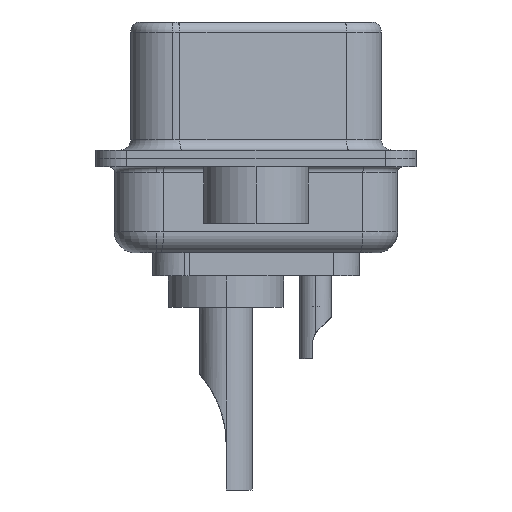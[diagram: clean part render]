
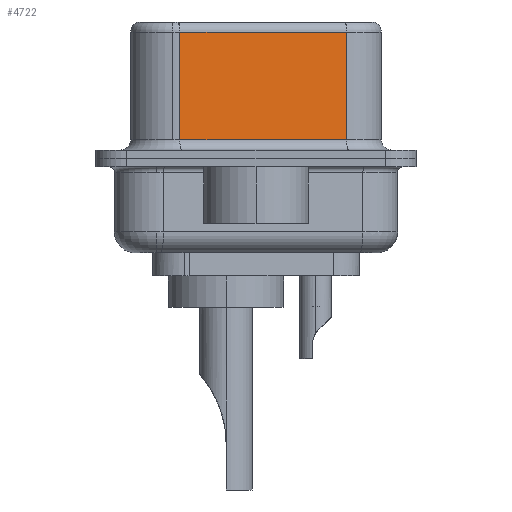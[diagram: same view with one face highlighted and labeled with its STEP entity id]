
A CAD part, left-side view. The second image highlights one B-rep face of the part: STEP entity #4722.
In plain terms, the highlighted planar face has unit normal (-0.985, -0.174, 0).
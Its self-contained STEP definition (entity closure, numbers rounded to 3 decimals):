
#138 = CARTESIAN_POINT ( 'NONE',  ( 5.132, -4.322, 6.02 ) ) ;
#170 = CARTESIAN_POINT ( 'NONE',  ( 3.73, 3.628, 6.02 ) ) ;
#595 = VECTOR ( 'NONE', #8259, 1000. ) ;
#1077 = CARTESIAN_POINT ( 'NONE',  ( 5.132, -4.322, 0.9 ) ) ;
#1236 = EDGE_CURVE ( 'NONE', #11570, #20293, #10309, .T. ) ;
#1310 = VECTOR ( 'NONE', #3485, 1000. ) ;
#3485 = DIRECTION ( 'NONE',  ( 0.174, -0.985, 0. ) ) ;
#4722 = ADVANCED_FACE ( 'NONE', ( #20140 ), #10655, .F. ) ;
#4771 = ORIENTED_EDGE ( 'NONE', *, *, #15640, .T. ) ;
#4964 = EDGE_CURVE ( 'NONE', #15760, #20293, #15509, .T. ) ;
#5144 = EDGE_LOOP ( 'NONE', ( #6338, #4771, #6441, #7594 ) ) ;
#5192 = DIRECTION ( 'NONE',  ( -0.174, 0.985, 0. ) ) ;
#5443 = DIRECTION ( 'NONE',  ( 0.985, 0.174, 0. ) ) ;
#5470 = CARTESIAN_POINT ( 'NONE',  ( 5.132, -4.322, 6.52 ) ) ;
#5629 = CARTESIAN_POINT ( 'NONE',  ( 3.73, 3.628, 0.9 ) ) ;
#5824 = VECTOR ( 'NONE', #13591, 1000. ) ;
#6338 = ORIENTED_EDGE ( 'NONE', *, *, #4964, .F. ) ;
#6441 = ORIENTED_EDGE ( 'NONE', *, *, #18506, .T. ) ;
#7594 = ORIENTED_EDGE ( 'NONE', *, *, #1236, .T. ) ;
#8259 = DIRECTION ( 'NONE',  ( -0.174, 0.985, 0. ) ) ;
#9566 = LINE ( 'NONE', #9988, #595 ) ;
#9988 = CARTESIAN_POINT ( 'NONE',  ( 5.132, -4.322, 6.02 ) ) ;
#10145 = CARTESIAN_POINT ( 'NONE',  ( 3.73, 3.628, 6.52 ) ) ;
#10268 = LINE ( 'NONE', #10145, #5824 ) ;
#10309 = LINE ( 'NONE', #1077, #1310 ) ;
#10655 = PLANE ( 'NONE',  #11308 ) ;
#10729 = CARTESIAN_POINT ( 'NONE',  ( 5.132, -4.322, 0.9 ) ) ;
#10806 = DIRECTION ( 'NONE',  ( 0., 0., -1. ) ) ;
#11045 = VECTOR ( 'NONE', #10806, 1000. ) ;
#11308 = AXIS2_PLACEMENT_3D ( 'NONE', #5470, #5443, #5192 ) ;
#11570 = VERTEX_POINT ( 'NONE', #5629 ) ;
#11736 = CARTESIAN_POINT ( 'NONE',  ( 5.132, -4.322, 6.52 ) ) ;
#13591 = DIRECTION ( 'NONE',  ( 0., 0., -1. ) ) ;
#15509 = LINE ( 'NONE', #11736, #11045 ) ;
#15640 = EDGE_CURVE ( 'NONE', #15760, #17871, #9566, .T. ) ;
#15760 = VERTEX_POINT ( 'NONE', #138 ) ;
#17871 = VERTEX_POINT ( 'NONE', #170 ) ;
#18506 = EDGE_CURVE ( 'NONE', #17871, #11570, #10268, .T. ) ;
#20140 = FACE_OUTER_BOUND ( 'NONE', #5144, .T. ) ;
#20293 = VERTEX_POINT ( 'NONE', #10729 ) ;
